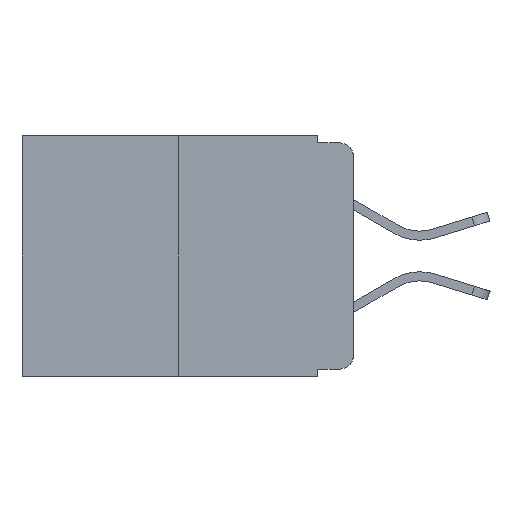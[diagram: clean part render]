
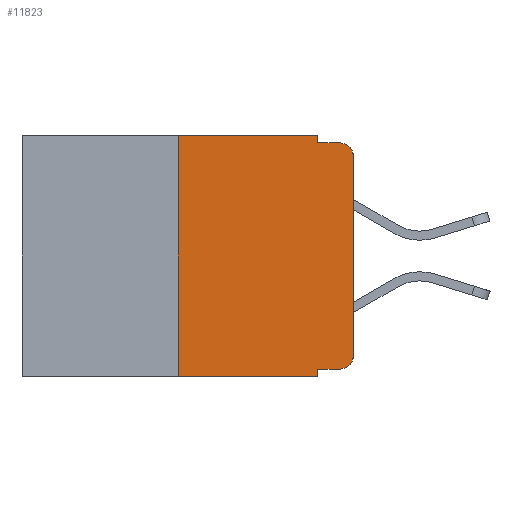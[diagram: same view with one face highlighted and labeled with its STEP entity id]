
A CAD part, left-side view. The second image highlights one B-rep face of the part: STEP entity #11823.
In plain terms, the highlighted planar face has unit normal (-1, 0, 0).
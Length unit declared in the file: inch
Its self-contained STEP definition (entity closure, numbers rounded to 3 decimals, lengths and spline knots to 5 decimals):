
#41 = EDGE_LOOP ( 'NONE', ( #8969, #11881, #6596, #14465, #15011, #13905, #13840, #2003, #6909, #7935 ) ) ;
#204 = LINE ( 'NONE', #4715, #12369 ) ;
#306 = VERTEX_POINT ( 'NONE', #7545 ) ;
#374 = LINE ( 'NONE', #3976, #929 ) ;
#389 = VERTEX_POINT ( 'NONE', #1179 ) ;
#449 = CARTESIAN_POINT ( 'NONE',  ( 0., 0.051, -0.333 ) ) ;
#582 = CARTESIAN_POINT ( 'NONE',  ( 0., 0.02, -0.313 ) ) ;
#624 = CARTESIAN_POINT ( 'NONE',  ( 0., 0.473, 0. ) ) ;
#929 = VECTOR ( 'NONE', #6346, 39.37008 ) ;
#1039 = LINE ( 'NONE', #15175, #11524 ) ;
#1084 = DIRECTION ( 'NONE',  ( 0., 0., 1. ) ) ;
#1176 = DIRECTION ( 'NONE',  ( 0., -1., 0. ) ) ;
#1179 = CARTESIAN_POINT ( 'NONE',  ( 0., 0., -0.03 ) ) ;
#1864 = DIRECTION ( 'NONE',  ( -1., 0., 0. ) ) ;
#2003 = ORIENTED_EDGE ( 'NONE', *, *, #12615, .F. ) ;
#2073 = VERTEX_POINT ( 'NONE', #13736 ) ;
#2661 = VECTOR ( 'NONE', #10410, 39.37008 ) ;
#2667 = VERTEX_POINT ( 'NONE', #6841 ) ;
#2939 = VECTOR ( 'NONE', #13848, 39.37008 ) ;
#2961 = EDGE_CURVE ( 'NONE', #12585, #2073, #6350, .T. ) ;
#3201 = VERTEX_POINT ( 'NONE', #14970 ) ;
#3300 = LINE ( 'NONE', #8067, #2939 ) ;
#3549 = AXIS2_PLACEMENT_3D ( 'NONE', #582, #13767, #10261 ) ;
#3976 = CARTESIAN_POINT ( 'NONE',  ( 0., 0.473, 0. ) ) ;
#3999 = CARTESIAN_POINT ( 'NONE',  ( 0., 0.051, -0.01 ) ) ;
#4007 = DIRECTION ( 'NONE',  ( 0., -1., 0. ) ) ;
#4355 = LINE ( 'NONE', #449, #9887 ) ;
#4550 = CARTESIAN_POINT ( 'NONE',  ( 0., 0.25, -0.343 ) ) ;
#4575 = CARTESIAN_POINT ( 'NONE',  ( 0., 0., -0.313 ) ) ;
#4715 = CARTESIAN_POINT ( 'NONE',  ( 0., 0.051, -0.01 ) ) ;
#4958 = LINE ( 'NONE', #13624, #13243 ) ;
#5498 = PLANE ( 'NONE',  #7594 ) ;
#6008 = EDGE_CURVE ( 'NONE', #15209, #12399, #204, .T. ) ;
#6295 = EDGE_CURVE ( 'NONE', #2073, #2667, #374, .T. ) ;
#6346 = DIRECTION ( 'NONE',  ( 0., -1., 0. ) ) ;
#6350 = LINE ( 'NONE', #14854, #2661 ) ;
#6596 = ORIENTED_EDGE ( 'NONE', *, *, #6008, .F. ) ;
#6674 = DIRECTION ( 'NONE',  ( 0., -1., 0. ) ) ;
#6841 = CARTESIAN_POINT ( 'NONE',  ( 0., 0.051, 0. ) ) ;
#6909 = ORIENTED_EDGE ( 'NONE', *, *, #13480, .T. ) ;
#7035 = EDGE_CURVE ( 'NONE', #389, #12399, #7731, .T. ) ;
#7249 = VERTEX_POINT ( 'NONE', #4575 ) ;
#7341 = AXIS2_PLACEMENT_3D ( 'NONE', #14841, #1864, #13799 ) ;
#7354 = LINE ( 'NONE', #12743, #12503 ) ;
#7509 = CARTESIAN_POINT ( 'NONE',  ( 0., 0.02, -0.01 ) ) ;
#7545 = CARTESIAN_POINT ( 'NONE',  ( 0., 0.02, -0.333 ) ) ;
#7594 = AXIS2_PLACEMENT_3D ( 'NONE', #624, #12557, #8896 ) ;
#7731 = CIRCLE ( 'NONE', #7341, 0.02 ) ;
#7935 = ORIENTED_EDGE ( 'NONE', *, *, #11267, .T. ) ;
#8067 = CARTESIAN_POINT ( 'NONE',  ( 0., 0.051, 0. ) ) ;
#8896 = DIRECTION ( 'NONE',  ( 0., 0., -1. ) ) ;
#8969 = ORIENTED_EDGE ( 'NONE', *, *, #9287, .T. ) ;
#9287 = EDGE_CURVE ( 'NONE', #7249, #389, #1039, .T. ) ;
#9387 = FACE_OUTER_BOUND ( 'NONE', #41, .T. ) ;
#9887 = VECTOR ( 'NONE', #4007, 39.37008 ) ;
#10261 = DIRECTION ( 'NONE',  ( 0., 0., -1. ) ) ;
#10410 = DIRECTION ( 'NONE',  ( 0., 0., 1. ) ) ;
#10780 = CARTESIAN_POINT ( 'NONE',  ( 0., 0.051, -0.343 ) ) ;
#11267 = EDGE_CURVE ( 'NONE', #306, #7249, #13470, .T. ) ;
#11524 = VECTOR ( 'NONE', #1084, 39.37008 ) ;
#11603 = DIRECTION ( 'NONE',  ( 0., 0., -1. ) ) ;
#11823 = ADVANCED_FACE ( 'NONE', ( #9387 ), #5498, .F. ) ;
#11881 = ORIENTED_EDGE ( 'NONE', *, *, #7035, .T. ) ;
#11935 = EDGE_CURVE ( 'NONE', #2667, #15209, #3300, .T. ) ;
#12369 = VECTOR ( 'NONE', #1176, 39.37008 ) ;
#12399 = VERTEX_POINT ( 'NONE', #7509 ) ;
#12503 = VECTOR ( 'NONE', #11603, 39.37008 ) ;
#12504 = EDGE_CURVE ( 'NONE', #12585, #12765, #4958, .T. ) ;
#12557 = DIRECTION ( 'NONE',  ( 1., 0., 0. ) ) ;
#12585 = VERTEX_POINT ( 'NONE', #4550 ) ;
#12615 = EDGE_CURVE ( 'NONE', #3201, #12765, #7354, .T. ) ;
#12743 = CARTESIAN_POINT ( 'NONE',  ( 0., 0.051, 0. ) ) ;
#12765 = VERTEX_POINT ( 'NONE', #10780 ) ;
#13243 = VECTOR ( 'NONE', #6674, 39.37008 ) ;
#13470 = CIRCLE ( 'NONE', #3549, 0.02 ) ;
#13480 = EDGE_CURVE ( 'NONE', #3201, #306, #4355, .T. ) ;
#13624 = CARTESIAN_POINT ( 'NONE',  ( 0., 0.473, -0.343 ) ) ;
#13736 = CARTESIAN_POINT ( 'NONE',  ( 0., 0.25, 0. ) ) ;
#13767 = DIRECTION ( 'NONE',  ( -1., 0., 0. ) ) ;
#13799 = DIRECTION ( 'NONE',  ( 0., 0., -1. ) ) ;
#13840 = ORIENTED_EDGE ( 'NONE', *, *, #12504, .T. ) ;
#13848 = DIRECTION ( 'NONE',  ( 0., 0., -1. ) ) ;
#13905 = ORIENTED_EDGE ( 'NONE', *, *, #2961, .F. ) ;
#14465 = ORIENTED_EDGE ( 'NONE', *, *, #11935, .F. ) ;
#14841 = CARTESIAN_POINT ( 'NONE',  ( 0., 0.02, -0.03 ) ) ;
#14854 = CARTESIAN_POINT ( 'NONE',  ( 0., 0.25, 0. ) ) ;
#14970 = CARTESIAN_POINT ( 'NONE',  ( 0., 0.051, -0.333 ) ) ;
#15011 = ORIENTED_EDGE ( 'NONE', *, *, #6295, .F. ) ;
#15175 = CARTESIAN_POINT ( 'NONE',  ( 0., 0., 0. ) ) ;
#15209 = VERTEX_POINT ( 'NONE', #3999 ) ;
